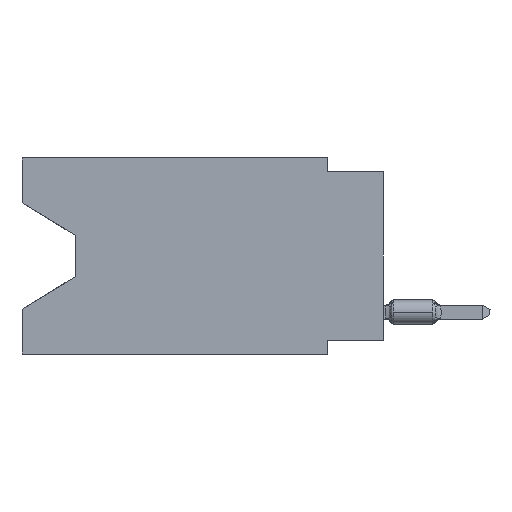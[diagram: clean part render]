
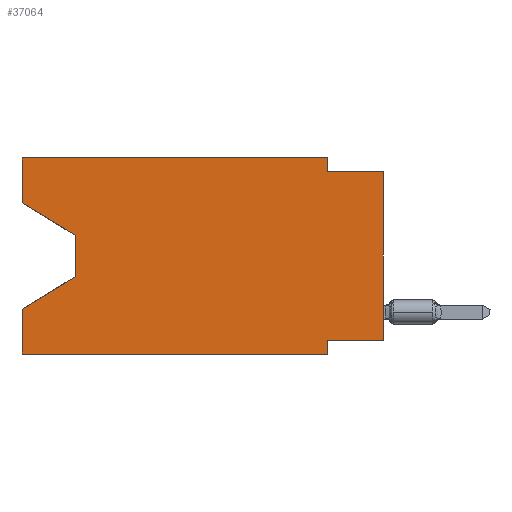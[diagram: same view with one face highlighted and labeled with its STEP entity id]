
A CAD part, left-side view. The second image highlights one B-rep face of the part: STEP entity #37064.
In plain terms, the highlighted planar face has unit normal (-1, 0, 0).
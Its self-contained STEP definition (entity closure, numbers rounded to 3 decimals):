
#10 = VERTEX_POINT ( 'NONE', #17065 ) ;
#48 = LINE ( 'NONE', #11041, #23857 ) ;
#98 = VERTEX_POINT ( 'NONE', #10144 ) ;
#293 = DIRECTION ( 'NONE',  ( 0., 0., -1. ) ) ;
#1061 = VERTEX_POINT ( 'NONE', #20542 ) ;
#1498 = DIRECTION ( 'NONE',  ( 0., 0., 1. ) ) ;
#1865 = ORIENTED_EDGE ( 'NONE', *, *, #33838, .F. ) ;
#2744 = DIRECTION ( 'NONE',  ( 0., -1., 0. ) ) ;
#4062 = VERTEX_POINT ( 'NONE', #47714 ) ;
#4214 = PLANE ( 'NONE',  #46514 ) ;
#4288 = VERTEX_POINT ( 'NONE', #18033 ) ;
#4419 = ORIENTED_EDGE ( 'NONE', *, *, #13222, .F. ) ;
#5510 = VECTOR ( 'NONE', #47674, 1000. ) ;
#5804 = VERTEX_POINT ( 'NONE', #24646 ) ;
#5913 = ORIENTED_EDGE ( 'NONE', *, *, #36625, .F. ) ;
#6992 = DIRECTION ( 'NONE',  ( 0., -1., 0. ) ) ;
#7848 = LINE ( 'NONE', #19882, #48681 ) ;
#8782 = CARTESIAN_POINT ( 'NONE',  ( 0., 16.383, 0. ) ) ;
#9103 = VECTOR ( 'NONE', #6992, 1000. ) ;
#9164 = CARTESIAN_POINT ( 'NONE',  ( 0., 16.383, 0. ) ) ;
#9759 = LINE ( 'NONE', #28452, #5510 ) ;
#10144 = CARTESIAN_POINT ( 'NONE',  ( 0., 2.54, -8.255 ) ) ;
#10233 = CARTESIAN_POINT ( 'NONE',  ( 0., 13.97, -5.385 ) ) ;
#10613 = VECTOR ( 'NONE', #2744, 1000. ) ;
#11041 = CARTESIAN_POINT ( 'NONE',  ( 0., 2.54, -8.89 ) ) ;
#11363 = VERTEX_POINT ( 'NONE', #17910 ) ;
#12648 = EDGE_CURVE ( 'NONE', #5804, #1061, #40198, .T. ) ;
#13222 = EDGE_CURVE ( 'NONE', #10, #5804, #44248, .T. ) ;
#13894 = CARTESIAN_POINT ( 'NONE',  ( 0., 16.383, -2.038 ) ) ;
#14176 = CARTESIAN_POINT ( 'NONE',  ( 0., 16.383, -8.89 ) ) ;
#14866 = ORIENTED_EDGE ( 'NONE', *, *, #16704, .F. ) ;
#15739 = VERTEX_POINT ( 'NONE', #13894 ) ;
#16704 = EDGE_CURVE ( 'NONE', #1061, #20845, #38229, .T. ) ;
#17065 = CARTESIAN_POINT ( 'NONE',  ( 0., 16.383, 0. ) ) ;
#17106 = CARTESIAN_POINT ( 'NONE',  ( 0., 16.383, 0. ) ) ;
#17126 = VERTEX_POINT ( 'NONE', #18213 ) ;
#17910 = CARTESIAN_POINT ( 'NONE',  ( 0., 16.383, -6.852 ) ) ;
#18033 = CARTESIAN_POINT ( 'NONE',  ( 0., 0., -8.255 ) ) ;
#18213 = CARTESIAN_POINT ( 'NONE',  ( 0., 13.97, -5.385 ) ) ;
#18252 = DIRECTION ( 'NONE',  ( 0., -1., 0. ) ) ;
#18584 = VECTOR ( 'NONE', #1498, 1000. ) ;
#18645 = VECTOR ( 'NONE', #49467, 1000. ) ;
#19553 = LINE ( 'NONE', #23373, #44899 ) ;
#19882 = CARTESIAN_POINT ( 'NONE',  ( 0., 16.383, 0. ) ) ;
#20394 = VECTOR ( 'NONE', #293, 1000. ) ;
#20482 = CARTESIAN_POINT ( 'NONE',  ( 0., 16.383, -8.89 ) ) ;
#20542 = CARTESIAN_POINT ( 'NONE',  ( 0., 2.54, -0.635 ) ) ;
#20845 = VERTEX_POINT ( 'NONE', #23708 ) ;
#22888 = CARTESIAN_POINT ( 'NONE',  ( 0., 0., -0.635 ) ) ;
#23373 = CARTESIAN_POINT ( 'NONE',  ( 0., 13.97, -3.505 ) ) ;
#23505 = VECTOR ( 'NONE', #25843, 1000. ) ;
#23624 = CARTESIAN_POINT ( 'NONE',  ( 0., 2.54, -8.89 ) ) ;
#23708 = CARTESIAN_POINT ( 'NONE',  ( 0., 0., -0.635 ) ) ;
#23857 = VECTOR ( 'NONE', #42551, 1000. ) ;
#24309 = CARTESIAN_POINT ( 'NONE',  ( 0., 2.54, 0. ) ) ;
#24397 = DIRECTION ( 'NONE',  ( 1., 0., 0. ) ) ;
#24646 = CARTESIAN_POINT ( 'NONE',  ( 0., 2.54, 0. ) ) ;
#24839 = LINE ( 'NONE', #10233, #23505 ) ;
#25843 = DIRECTION ( 'NONE',  ( 0., 0.855, -0.519 ) ) ;
#26203 = LINE ( 'NONE', #14176, #47078 ) ;
#28073 = DIRECTION ( 'NONE',  ( 0., 0., 1. ) ) ;
#28452 = CARTESIAN_POINT ( 'NONE',  ( 0., 16.383, -2.038 ) ) ;
#29284 = DIRECTION ( 'NONE',  ( 0., 0., 1. ) ) ;
#29367 = ORIENTED_EDGE ( 'NONE', *, *, #39016, .T. ) ;
#29544 = LINE ( 'NONE', #49746, #42293 ) ;
#31229 = EDGE_CURVE ( 'NONE', #15739, #4062, #9759, .T. ) ;
#31859 = DIRECTION ( 'NONE',  ( 0., 0., -1. ) ) ;
#32419 = ORIENTED_EDGE ( 'NONE', *, *, #31229, .T. ) ;
#33838 = EDGE_CURVE ( 'NONE', #49766, #11363, #36564, .T. ) ;
#35189 = DIRECTION ( 'NONE',  ( 0., 0., -1. ) ) ;
#36564 = LINE ( 'NONE', #17106, #18584 ) ;
#36625 = EDGE_CURVE ( 'NONE', #4288, #98, #37931, .T. ) ;
#37064 = ADVANCED_FACE ( 'NONE', ( #43852 ), #4214, .F. ) ;
#37429 = CARTESIAN_POINT ( 'NONE',  ( 0., 0., -8.255 ) ) ;
#37499 = EDGE_CURVE ( 'NONE', #17126, #11363, #24839, .T. ) ;
#37931 = LINE ( 'NONE', #37429, #18645 ) ;
#38229 = LINE ( 'NONE', #22888, #9103 ) ;
#39016 = EDGE_CURVE ( 'NONE', #4062, #17126, #19553, .T. ) ;
#39878 = EDGE_CURVE ( 'NONE', #15739, #10, #7848, .T. ) ;
#40198 = LINE ( 'NONE', #24309, #20394 ) ;
#41772 = ORIENTED_EDGE ( 'NONE', *, *, #39878, .F. ) ;
#41834 = ORIENTED_EDGE ( 'NONE', *, *, #45263, .F. ) ;
#42293 = VECTOR ( 'NONE', #29284, 1000. ) ;
#42551 = DIRECTION ( 'NONE',  ( 0., 0., -1. ) ) ;
#42861 = EDGE_LOOP ( 'NONE', ( #32419, #29367, #44646, #1865, #44484, #41834, #5913, #44316, #14866, #46349, #4419, #41772 ) ) ;
#43852 = FACE_OUTER_BOUND ( 'NONE', #42861, .T. ) ;
#44248 = LINE ( 'NONE', #9164, #10613 ) ;
#44316 = ORIENTED_EDGE ( 'NONE', *, *, #47776, .T. ) ;
#44484 = ORIENTED_EDGE ( 'NONE', *, *, #47781, .T. ) ;
#44646 = ORIENTED_EDGE ( 'NONE', *, *, #37499, .T. ) ;
#44899 = VECTOR ( 'NONE', #35189, 1000. ) ;
#45263 = EDGE_CURVE ( 'NONE', #98, #46277, #48, .T. ) ;
#46277 = VERTEX_POINT ( 'NONE', #23624 ) ;
#46349 = ORIENTED_EDGE ( 'NONE', *, *, #12648, .F. ) ;
#46514 = AXIS2_PLACEMENT_3D ( 'NONE', #8782, #24397, #31859 ) ;
#47078 = VECTOR ( 'NONE', #18252, 1000. ) ;
#47674 = DIRECTION ( 'NONE',  ( 0., -0.855, -0.519 ) ) ;
#47714 = CARTESIAN_POINT ( 'NONE',  ( 0., 13.97, -3.505 ) ) ;
#47776 = EDGE_CURVE ( 'NONE', #4288, #20845, #29544, .T. ) ;
#47781 = EDGE_CURVE ( 'NONE', #49766, #46277, #26203, .T. ) ;
#48681 = VECTOR ( 'NONE', #28073, 1000. ) ;
#49467 = DIRECTION ( 'NONE',  ( 0., 1., 0. ) ) ;
#49746 = CARTESIAN_POINT ( 'NONE',  ( 0., 0., 0. ) ) ;
#49766 = VERTEX_POINT ( 'NONE', #20482 ) ;
